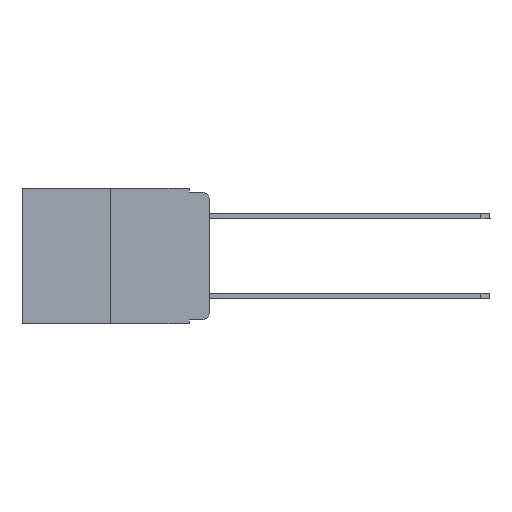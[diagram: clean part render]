
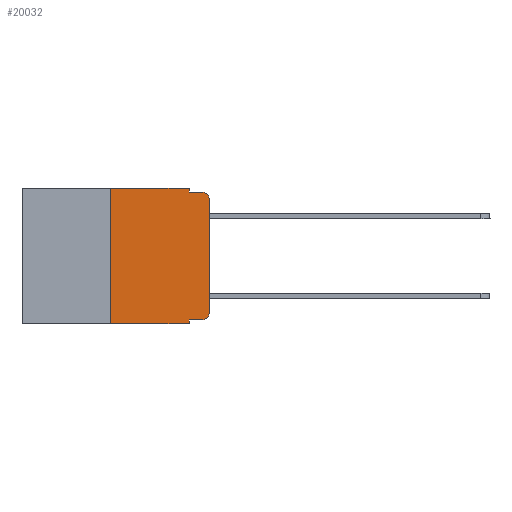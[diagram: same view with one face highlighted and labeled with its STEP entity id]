
A CAD part, left-side view. The second image highlights one B-rep face of the part: STEP entity #20032.
In plain terms, the highlighted planar face has unit normal (-1, 0, 0).
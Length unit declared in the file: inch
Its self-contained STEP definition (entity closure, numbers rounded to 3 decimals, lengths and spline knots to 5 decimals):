
#25 = DIRECTION ( 'NONE',  ( 0., -1., 0. ) ) ;
#331 = EDGE_CURVE ( 'NONE', #11065, #12360, #3313, .T. ) ;
#1009 = DIRECTION ( 'NONE',  ( 0., 0., -1. ) ) ;
#1246 = LINE ( 'NONE', #9504, #7923 ) ;
#1403 = VERTEX_POINT ( 'NONE', #9734 ) ;
#2365 = VERTEX_POINT ( 'NONE', #17846 ) ;
#2436 = LINE ( 'NONE', #13905, #7968 ) ;
#3094 = CARTESIAN_POINT ( 'NONE',  ( 0., 0.25, 0. ) ) ;
#3313 = CIRCLE ( 'NONE', #18022, 0.02 ) ;
#4243 = VERTEX_POINT ( 'NONE', #23645 ) ;
#4551 = CARTESIAN_POINT ( 'NONE',  ( 0., 0.25, 0. ) ) ;
#5369 = CARTESIAN_POINT ( 'NONE',  ( 0., 0.02, -0.01 ) ) ;
#5387 = ORIENTED_EDGE ( 'NONE', *, *, #18954, .F. ) ;
#5864 = VERTEX_POINT ( 'NONE', #18958 ) ;
#6082 = VERTEX_POINT ( 'NONE', #21767 ) ;
#6185 = ORIENTED_EDGE ( 'NONE', *, *, #11110, .T. ) ;
#6984 = EDGE_CURVE ( 'NONE', #2365, #6082, #16031, .T. ) ;
#7088 = CARTESIAN_POINT ( 'NONE',  ( 0., 0.25, -0.343 ) ) ;
#7664 = DIRECTION ( 'NONE',  ( 0., -1., 0. ) ) ;
#7884 = DIRECTION ( 'NONE',  ( 0., 0., -1. ) ) ;
#7923 = VECTOR ( 'NONE', #7664, 39.37008 ) ;
#7968 = VECTOR ( 'NONE', #23066, 39.37008 ) ;
#9256 = CARTESIAN_POINT ( 'NONE',  ( 0., 0.02, -0.313 ) ) ;
#9490 = CARTESIAN_POINT ( 'NONE',  ( 0., 0.051, 0. ) ) ;
#9504 = CARTESIAN_POINT ( 'NONE',  ( 0., 0.473, 0. ) ) ;
#9656 = LINE ( 'NONE', #14835, #14000 ) ;
#9734 = CARTESIAN_POINT ( 'NONE',  ( 0., 0.051, -0.343 ) ) ;
#10000 = DIRECTION ( 'NONE',  ( -1., 0., 0. ) ) ;
#10307 = LINE ( 'NONE', #12100, #18459 ) ;
#10392 = ORIENTED_EDGE ( 'NONE', *, *, #23030, .T. ) ;
#10612 = CARTESIAN_POINT ( 'NONE',  ( 0., 0., 0. ) ) ;
#10799 = LINE ( 'NONE', #4551, #17205 ) ;
#10895 = EDGE_CURVE ( 'NONE', #6082, #11065, #11989, .T. ) ;
#10937 = VERTEX_POINT ( 'NONE', #3094 ) ;
#10974 = CARTESIAN_POINT ( 'NONE',  ( 0., 0.473, 0. ) ) ;
#11065 = VERTEX_POINT ( 'NONE', #12896 ) ;
#11110 = EDGE_CURVE ( 'NONE', #5864, #2365, #9656, .T. ) ;
#11190 = FACE_OUTER_BOUND ( 'NONE', #12255, .T. ) ;
#11247 = EDGE_CURVE ( 'NONE', #19691, #12360, #2436, .T. ) ;
#11918 = EDGE_CURVE ( 'NONE', #14213, #10937, #10799, .T. ) ;
#11989 = LINE ( 'NONE', #10612, #17255 ) ;
#12100 = CARTESIAN_POINT ( 'NONE',  ( 0., 0.051, 0. ) ) ;
#12159 = DIRECTION ( 'NONE',  ( 0., 0., 1. ) ) ;
#12190 = LINE ( 'NONE', #22544, #20860 ) ;
#12255 = EDGE_LOOP ( 'NONE', ( #12622, #14348, #22594, #5387, #22413, #17915, #10392, #21899, #6185, #18553 ) ) ;
#12360 = VERTEX_POINT ( 'NONE', #5369 ) ;
#12622 = ORIENTED_EDGE ( 'NONE', *, *, #10895, .T. ) ;
#12877 = LINE ( 'NONE', #9490, #17241 ) ;
#12896 = CARTESIAN_POINT ( 'NONE',  ( 0., 0., -0.03 ) ) ;
#13326 = DIRECTION ( 'NONE',  ( 0., -1., 0. ) ) ;
#13877 = CARTESIAN_POINT ( 'NONE',  ( 0., 0.02, -0.03 ) ) ;
#13905 = CARTESIAN_POINT ( 'NONE',  ( 0., 0.051, -0.01 ) ) ;
#14000 = VECTOR ( 'NONE', #25, 39.37008 ) ;
#14213 = VERTEX_POINT ( 'NONE', #7088 ) ;
#14348 = ORIENTED_EDGE ( 'NONE', *, *, #331, .T. ) ;
#14435 = DIRECTION ( 'NONE',  ( 0., 0., -1. ) ) ;
#14835 = CARTESIAN_POINT ( 'NONE',  ( 0., 0.051, -0.333 ) ) ;
#15757 = DIRECTION ( 'NONE',  ( 0., 0., -1. ) ) ;
#16031 = CIRCLE ( 'NONE', #23577, 0.02 ) ;
#17205 = VECTOR ( 'NONE', #21485, 39.37008 ) ;
#17241 = VECTOR ( 'NONE', #7884, 39.37008 ) ;
#17255 = VECTOR ( 'NONE', #12159, 39.37008 ) ;
#17846 = CARTESIAN_POINT ( 'NONE',  ( 0., 0.02, -0.333 ) ) ;
#17915 = ORIENTED_EDGE ( 'NONE', *, *, #11918, .F. ) ;
#18022 = AXIS2_PLACEMENT_3D ( 'NONE', #13877, #10000, #15757 ) ;
#18459 = VECTOR ( 'NONE', #1009, 39.37008 ) ;
#18553 = ORIENTED_EDGE ( 'NONE', *, *, #6984, .T. ) ;
#18954 = EDGE_CURVE ( 'NONE', #4243, #19691, #12877, .T. ) ;
#18958 = CARTESIAN_POINT ( 'NONE',  ( 0., 0.051, -0.333 ) ) ;
#19691 = VERTEX_POINT ( 'NONE', #23200 ) ;
#20032 = ADVANCED_FACE ( 'NONE', ( #11190 ), #22225, .F. ) ;
#20140 = DIRECTION ( 'NONE',  ( 1., 0., 0. ) ) ;
#20392 = EDGE_CURVE ( 'NONE', #5864, #1403, #10307, .T. ) ;
#20860 = VECTOR ( 'NONE', #13326, 39.37008 ) ;
#21485 = DIRECTION ( 'NONE',  ( 0., 0., 1. ) ) ;
#21708 = EDGE_CURVE ( 'NONE', #10937, #4243, #1246, .T. ) ;
#21767 = CARTESIAN_POINT ( 'NONE',  ( 0., 0., -0.313 ) ) ;
#21899 = ORIENTED_EDGE ( 'NONE', *, *, #20392, .F. ) ;
#21982 = DIRECTION ( 'NONE',  ( 0., 0., -1. ) ) ;
#22195 = DIRECTION ( 'NONE',  ( -1., 0., 0. ) ) ;
#22225 = PLANE ( 'NONE',  #23938 ) ;
#22413 = ORIENTED_EDGE ( 'NONE', *, *, #21708, .F. ) ;
#22544 = CARTESIAN_POINT ( 'NONE',  ( 0., 0.473, -0.343 ) ) ;
#22594 = ORIENTED_EDGE ( 'NONE', *, *, #11247, .F. ) ;
#23030 = EDGE_CURVE ( 'NONE', #14213, #1403, #12190, .T. ) ;
#23066 = DIRECTION ( 'NONE',  ( 0., -1., 0. ) ) ;
#23200 = CARTESIAN_POINT ( 'NONE',  ( 0., 0.051, -0.01 ) ) ;
#23577 = AXIS2_PLACEMENT_3D ( 'NONE', #9256, #22195, #14435 ) ;
#23645 = CARTESIAN_POINT ( 'NONE',  ( 0., 0.051, 0. ) ) ;
#23938 = AXIS2_PLACEMENT_3D ( 'NONE', #10974, #20140, #21982 ) ;
